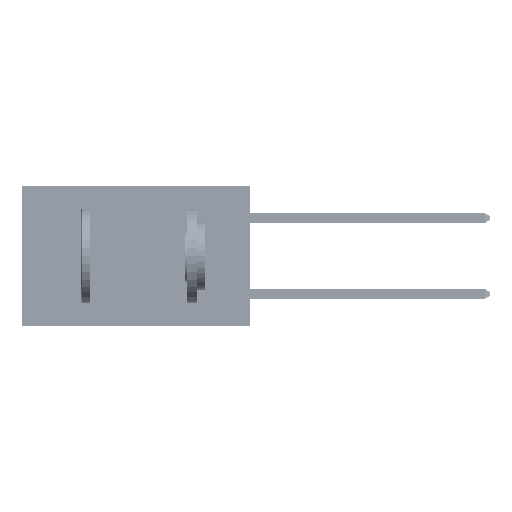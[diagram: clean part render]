
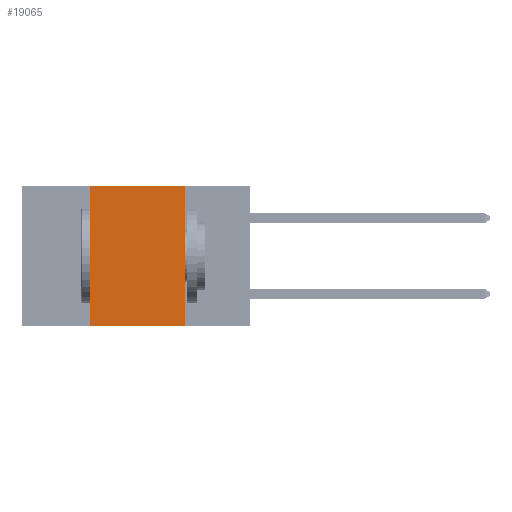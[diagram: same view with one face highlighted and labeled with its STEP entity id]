
A CAD part, left-side view. The second image highlights one B-rep face of the part: STEP entity #19065.
In plain terms, the highlighted planar face has unit normal (-1, 0, 0).
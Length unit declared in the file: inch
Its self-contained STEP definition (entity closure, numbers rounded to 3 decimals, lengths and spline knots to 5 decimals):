
#217 = VERTEX_POINT ( 'NONE', #18406 ) ;
#2354 = CARTESIAN_POINT ( 'NONE',  ( 0., 0.6, 0. ) ) ;
#2701 = CARTESIAN_POINT ( 'NONE',  ( 0., 0.17, -0.37 ) ) ;
#5406 = CARTESIAN_POINT ( 'NONE',  ( 0., 0.17, 0. ) ) ;
#6083 = EDGE_CURVE ( 'NONE', #20473, #18599, #31356, .T. ) ;
#9094 = DIRECTION ( 'NONE',  ( 0., 0., 1. ) ) ;
#9579 = LINE ( 'NONE', #17502, #51611 ) ;
#10299 = EDGE_CURVE ( 'NONE', #16034, #217, #9579, .T. ) ;
#12313 = AXIS2_PLACEMENT_3D ( 'NONE', #49489, #25482, #33871 ) ;
#13013 = ORIENTED_EDGE ( 'NONE', *, *, #21691, .T. ) ;
#13099 = ORIENTED_EDGE ( 'NONE', *, *, #42009, .F. ) ;
#16034 = VERTEX_POINT ( 'NONE', #17549 ) ;
#17334 = EDGE_LOOP ( 'NONE', ( #43591, #13099, #34868, #13013 ) ) ;
#17502 = CARTESIAN_POINT ( 'NONE',  ( 0., 0.42, 0. ) ) ;
#17549 = CARTESIAN_POINT ( 'NONE',  ( 0., 0.42, -0.37 ) ) ;
#18406 = CARTESIAN_POINT ( 'NONE',  ( 0., 0.42, 0. ) ) ;
#18599 = VERTEX_POINT ( 'NONE', #2701 ) ;
#19065 = ADVANCED_FACE ( 'NONE', ( #41419 ), #37385, .F. ) ;
#20473 = VERTEX_POINT ( 'NONE', #26001 ) ;
#21104 = LINE ( 'NONE', #46835, #38691 ) ;
#21691 = EDGE_CURVE ( 'NONE', #16034, #18599, #21104, .T. ) ;
#22102 = DIRECTION ( 'NONE',  ( 0., -1., 0. ) ) ;
#25482 = DIRECTION ( 'NONE',  ( 1., 0., 0. ) ) ;
#26001 = CARTESIAN_POINT ( 'NONE',  ( 0., 0.17, 0. ) ) ;
#26595 = DIRECTION ( 'NONE',  ( 0., -1., 0. ) ) ;
#29788 = DIRECTION ( 'NONE',  ( 0., 0., -1. ) ) ;
#30528 = LINE ( 'NONE', #2354, #32390 ) ;
#31356 = LINE ( 'NONE', #5406, #39542 ) ;
#32390 = VECTOR ( 'NONE', #26595, 39.37008 ) ;
#33871 = DIRECTION ( 'NONE',  ( 0., 0., -1. ) ) ;
#34868 = ORIENTED_EDGE ( 'NONE', *, *, #10299, .F. ) ;
#37385 = PLANE ( 'NONE',  #12313 ) ;
#38691 = VECTOR ( 'NONE', #22102, 39.37008 ) ;
#39542 = VECTOR ( 'NONE', #29788, 39.37008 ) ;
#41419 = FACE_OUTER_BOUND ( 'NONE', #17334, .T. ) ;
#42009 = EDGE_CURVE ( 'NONE', #217, #20473, #30528, .T. ) ;
#43591 = ORIENTED_EDGE ( 'NONE', *, *, #6083, .F. ) ;
#46835 = CARTESIAN_POINT ( 'NONE',  ( 0., 0.6, -0.37 ) ) ;
#49489 = CARTESIAN_POINT ( 'NONE',  ( 0., 0.6, 0. ) ) ;
#51611 = VECTOR ( 'NONE', #9094, 39.37008 ) ;
